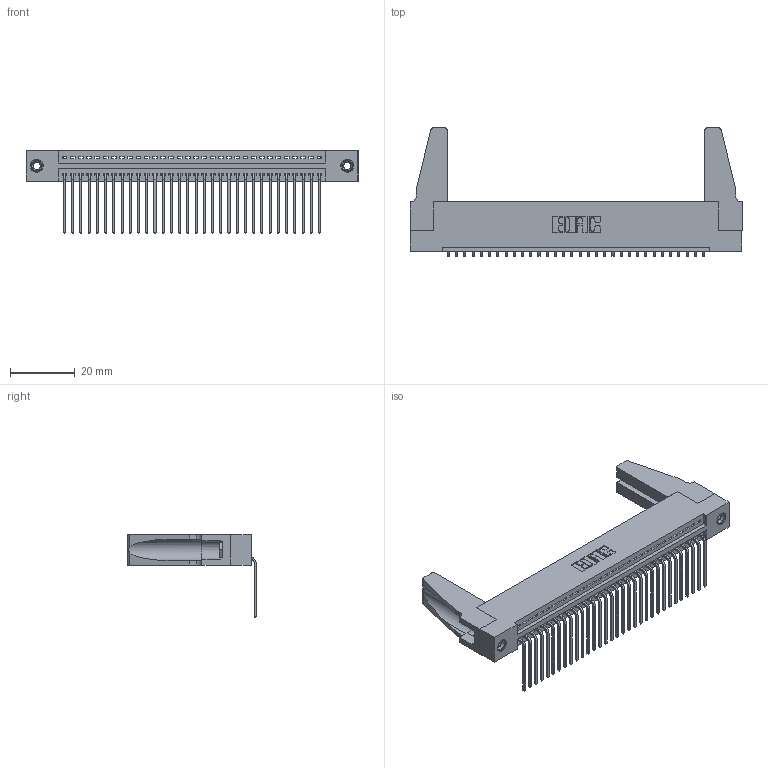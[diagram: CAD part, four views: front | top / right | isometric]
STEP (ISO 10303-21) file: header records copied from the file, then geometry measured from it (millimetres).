
FILE_DESCRIPTION (( 'STEP AP203' ), '1' );
FILE_NAME ('395-032-559-188.STEP', '2019-10-19T15:01:04', ( '' ), ( '' ), 'SwSTEP 2.0', 'SolidWorks 2016', '' );
FILE_SCHEMA (( 'CONFIG_CONTROL_DESIGN' ));
Length unit declared in the file: inch
Products named in the file (5): 345 Part_Flush Mounting Lugs - 0.156 Dia-TH; 345-220-078_345-220-088; 345-292-001_558 559 Tail - 1; 395-032-559-188; 345-250-001_345-250-001-102
Assembly tree (37 placements, depth 2):
  395-032-559-188
    345 Part_Flush Mounting Lugs - 0.156 Dia-TH
    345-292-001_558 559 Tail - 1  x32
    345-250-001_345-250-001-102  x2
    345-220-078_345-220-088  x2
Bounding box: 102.51 x 39.61 x 25.53 mm (x, y, z)
Volume: 13014.1 mm3; surface area: 16592.2 mm2
Topology: 37 solids, 37 shells, 2170 faces, 6479 edges, 4266 vertices
Faces by surface type: plane 1496, cylinder 658, cone 12, torus 4
Entity records: 27662 total; most frequent: CARTESIAN_POINT 4782, ORIENTED_EDGE 4708, DIRECTION 4198, EDGE_CURVE 2354, VECTOR 2052, LINE 2052, VERTEX_POINT 1562, AXIS2_PLACEMENT_3D 1073
